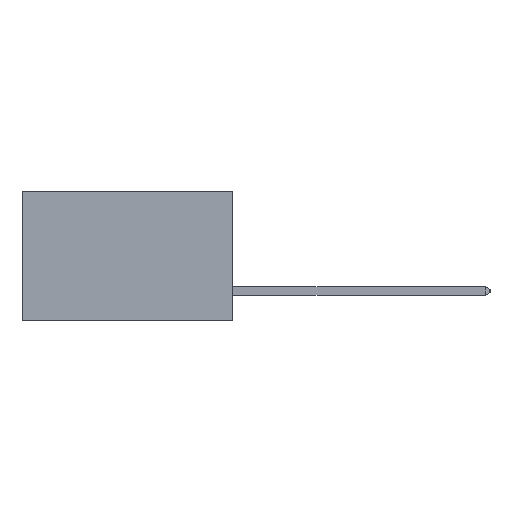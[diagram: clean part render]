
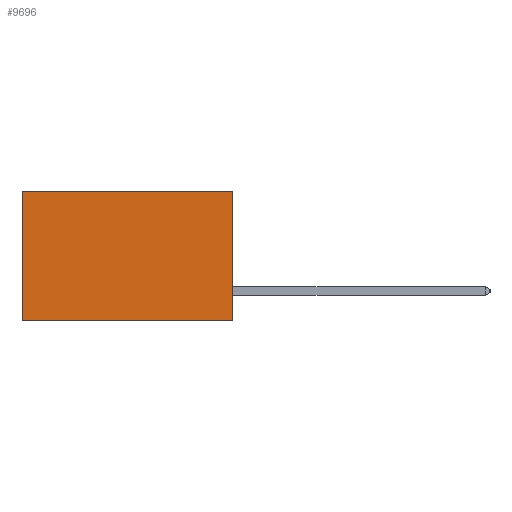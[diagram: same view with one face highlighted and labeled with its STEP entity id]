
A CAD part, left-side view. The second image highlights one B-rep face of the part: STEP entity #9696.
In plain terms, the highlighted planar face has unit normal (-1, 0, 0).
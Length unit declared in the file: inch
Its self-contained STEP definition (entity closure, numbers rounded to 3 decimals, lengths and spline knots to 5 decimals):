
#143 = CARTESIAN_POINT ( 'NONE',  ( 0.2875, 0., -0.37 ) ) ;
#1440 = CARTESIAN_POINT ( 'NONE',  ( 0.2875, 0., 0. ) ) ;
#1671 = CARTESIAN_POINT ( 'NONE',  ( 0.2875, 0., -0.37 ) ) ;
#1710 = VERTEX_POINT ( 'NONE', #8065 ) ;
#2558 = LINE ( 'NONE', #3495, #13121 ) ;
#2919 = ORIENTED_EDGE ( 'NONE', *, *, #7851, .T. ) ;
#3495 = CARTESIAN_POINT ( 'NONE',  ( 0.2875, 0., 0. ) ) ;
#3909 = ORIENTED_EDGE ( 'NONE', *, *, #12855, .F. ) ;
#4284 = EDGE_CURVE ( 'NONE', #9408, #15988, #8981, .T. ) ;
#6193 = PLANE ( 'NONE',  #14215 ) ;
#6350 = ORIENTED_EDGE ( 'NONE', *, *, #11629, .T. ) ;
#7117 = VECTOR ( 'NONE', #8565, 39.37008 ) ;
#7499 = DIRECTION ( 'NONE',  ( 0., 1., 0. ) ) ;
#7851 = EDGE_CURVE ( 'NONE', #9408, #1710, #2558, .T. ) ;
#7881 = VERTEX_POINT ( 'NONE', #8876 ) ;
#8065 = CARTESIAN_POINT ( 'NONE',  ( 0.2875, 0.6, 0. ) ) ;
#8565 = DIRECTION ( 'NONE',  ( 0., 0., -1. ) ) ;
#8826 = DIRECTION ( 'NONE',  ( 0., 0., -1. ) ) ;
#8876 = CARTESIAN_POINT ( 'NONE',  ( 0.2875, 0.6, -0.37 ) ) ;
#8981 = LINE ( 'NONE', #10226, #16520 ) ;
#9147 = EDGE_LOOP ( 'NONE', ( #6350, #3909, #12131, #2919 ) ) ;
#9408 = VERTEX_POINT ( 'NONE', #1440 ) ;
#9696 = ADVANCED_FACE ( 'NONE', ( #11297 ), #6193, .F. ) ;
#10170 = DIRECTION ( 'NONE',  ( 0., 0., -1. ) ) ;
#10226 = CARTESIAN_POINT ( 'NONE',  ( 0.2875, 0., 0. ) ) ;
#10622 = LINE ( 'NONE', #13685, #7117 ) ;
#11085 = DIRECTION ( 'NONE',  ( 0., 1., 0. ) ) ;
#11297 = FACE_OUTER_BOUND ( 'NONE', #9147, .T. ) ;
#11629 = EDGE_CURVE ( 'NONE', #1710, #7881, #10622, .T. ) ;
#12131 = ORIENTED_EDGE ( 'NONE', *, *, #4284, .F. ) ;
#12855 = EDGE_CURVE ( 'NONE', #15988, #7881, #13130, .T. ) ;
#13121 = VECTOR ( 'NONE', #7499, 39.37008 ) ;
#13130 = LINE ( 'NONE', #143, #16823 ) ;
#13685 = CARTESIAN_POINT ( 'NONE',  ( 0.2875, 0.6, 0. ) ) ;
#14215 = AXIS2_PLACEMENT_3D ( 'NONE', #15198, #16436, #8826 ) ;
#15198 = CARTESIAN_POINT ( 'NONE',  ( 0.2875, 0., 0. ) ) ;
#15988 = VERTEX_POINT ( 'NONE', #1671 ) ;
#16436 = DIRECTION ( 'NONE',  ( 1., 0., 0. ) ) ;
#16520 = VECTOR ( 'NONE', #10170, 39.37008 ) ;
#16823 = VECTOR ( 'NONE', #11085, 39.37008 ) ;
